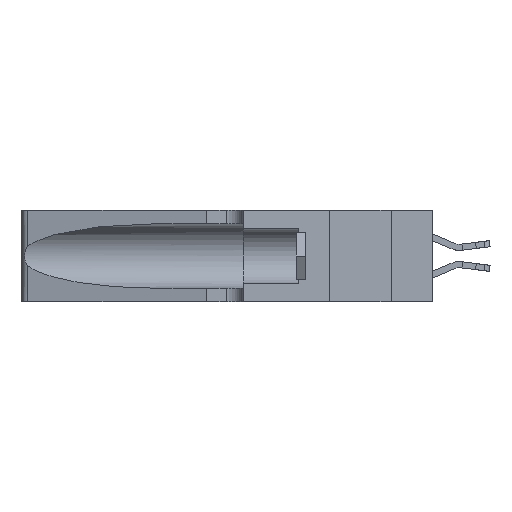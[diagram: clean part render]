
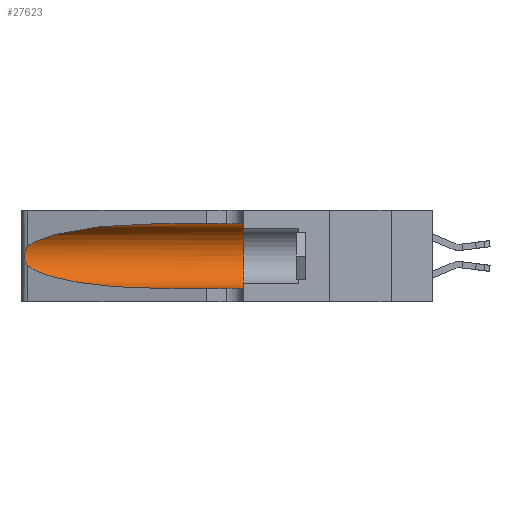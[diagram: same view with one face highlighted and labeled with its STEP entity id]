
A CAD part, left-side view. The second image highlights one B-rep face of the part: STEP entity #27623.
In plain terms, the highlighted cylindrical face has radius 3.308 mm (diameter 6.617 mm), a partial arc.
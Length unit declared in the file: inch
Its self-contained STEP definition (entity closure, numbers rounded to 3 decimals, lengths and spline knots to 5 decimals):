
#132 = CARTESIAN_POINT ( 'NONE',  ( 0.18966, 0.96281, 0.31525 ) ) ;
#293 = CARTESIAN_POINT ( 'NONE',  ( 0.1305, 0.35, 0.05475 ) ) ;
#329 = DIRECTION ( 'NONE',  ( 0., 1., 0. ) ) ;
#581 = B_SPLINE_CURVE_WITH_KNOTS ( 'NONE', 3,
 ( #30651, #11926, #3813, #22719, #6568, #25376, #9314, #28063, #12038, #30769, #14744, #33465, #17447, #1171 ),
 .UNSPECIFIED., .F., .F.,
 ( 4, 2, 2, 2, 2, 2, 4 ),
 ( 0., 0.00027, 0.00053, 0.00107, 0.0016, 0.00187, 0.00214 ),
 .UNSPECIFIED. ) ;
#1171 = CARTESIAN_POINT ( 'NONE',  ( 0.25487, 1.22718, 0.14631 ) ) ;
#1228 = ORIENTED_EDGE ( 'NONE', *, *, #17873, .T. ) ;
#1542 = EDGE_CURVE ( 'NONE', #30085, #18338, #31185, .T. ) ;
#2162 = LINE ( 'NONE', #15308, #22904 ) ;
#2334 = EDGE_CURVE ( 'NONE', #8358, #18338, #21103, .T. ) ;
#2861 = CARTESIAN_POINT ( 'NONE',  ( 0.25487, 1.22718, 0.14631 ) ) ;
#3148 = ORIENTED_EDGE ( 'NONE', *, *, #9684, .T. ) ;
#3813 = CARTESIAN_POINT ( 'NONE',  ( 0.25639, 1.23184, 0.21858 ) ) ;
#4668 = DIRECTION ( 'NONE',  ( 0., -1., 0. ) ) ;
#5190 = DIRECTION ( 'NONE',  ( 0., -1., 0. ) ) ;
#6568 = CARTESIAN_POINT ( 'NONE',  ( 0.25854, 1.2359, 0.20912 ) ) ;
#6579 = CARTESIAN_POINT ( 'NONE',  ( 0.1305, 0.72297, 0.31525 ) ) ;
#7106 = EDGE_CURVE ( 'NONE', #12279, #8358, #2162, .T. ) ;
#7494 = ORIENTED_EDGE ( 'NONE', *, *, #7106, .F. ) ;
#8358 = VERTEX_POINT ( 'NONE', #23224 ) ;
#8419 = CARTESIAN_POINT ( 'NONE',  ( 0.2373, 1.15595, 0.28018 ) ) ;
#9314 = CARTESIAN_POINT ( 'NONE',  ( 0.26075, 1.23896, 0.19203 ) ) ;
#9684 = EDGE_CURVE ( 'NONE', #25313, #30085, #19503, .T. ) ;
#9974 = ORIENTED_EDGE ( 'NONE', *, *, #33260, .T. ) ;
#10244 = ORIENTED_EDGE ( 'NONE', *, *, #1542, .T. ) ;
#11926 = CARTESIAN_POINT ( 'NONE',  ( 0.25555, 1.22994, 0.2215 ) ) ;
#12038 = CARTESIAN_POINT ( 'NONE',  ( 0.26017, 1.23833, 0.17102 ) ) ;
#12279 = VERTEX_POINT ( 'NONE', #6579 ) ;
#12888 = CARTESIAN_POINT ( 'NONE',  ( 0.1305, 1.61858, 0.185 ) ) ;
#13805 = ORIENTED_EDGE ( 'NONE', *, *, #2334, .F. ) ;
#14398 = CARTESIAN_POINT ( 'NONE',  ( 0.1305, 0.72297, 0.05475 ) ) ;
#14744 = CARTESIAN_POINT ( 'NONE',  ( 0.25789, 1.23486, 0.15765 ) ) ;
#15308 = CARTESIAN_POINT ( 'NONE',  ( 0.1305, 1.61858, 0.31525 ) ) ;
#16062 = AXIS2_PLACEMENT_3D ( 'NONE', #12888, #4668, #28899 ) ;
#16620 = CARTESIAN_POINT ( 'NONE',  ( 0.1305, 0.35, 0.185 ) ) ;
#16964 = VECTOR ( 'NONE', #5190, 39.37008 ) ;
#17383 = CARTESIAN_POINT ( 'NONE',  ( 0.2373, 1.15595, 0.08982 ) ) ;
#17447 = CARTESIAN_POINT ( 'NONE',  ( 0.25555, 1.22993, 0.14849 ) ) ;
#17873 = EDGE_CURVE ( 'NONE', #28362, #25313, #581, .T. ) ;
#18020 = DIRECTION ( 'NONE',  ( 0., -1., 0. ) ) ;
#18338 = VERTEX_POINT ( 'NONE', #293 ) ;
#19322 = DIRECTION ( 'NONE',  ( 0., 0., 1. ) ) ;
#19503 =( BOUNDED_CURVE ( )  B_SPLINE_CURVE ( 3, ( #20062, #17383, #33392, #22762 ),
 .UNSPECIFIED., .F., .F. ) 
 B_SPLINE_CURVE_WITH_KNOTS ( ( 4, 4 ),
 ( 3.44316, 4.71239 ),
 .UNSPECIFIED. ) 
 CURVE ( )  GEOMETRIC_REPRESENTATION_ITEM ( )  RATIONAL_B_SPLINE_CURVE ( ( 1., 0.87, 0.87, 1. ) ) 
 REPRESENTATION_ITEM ( '' )  );
#19615 = AXIS2_PLACEMENT_3D ( 'NONE', #16620, #329, #19322 ) ;
#20062 = CARTESIAN_POINT ( 'NONE',  ( 0.25487, 1.22718, 0.14631 ) ) ;
#20161 = FACE_OUTER_BOUND ( 'NONE', #24514, .T. ) ;
#21103 = CIRCLE ( 'NONE', #19615, 0.13025 ) ;
#22719 = CARTESIAN_POINT ( 'NONE',  ( 0.25787, 1.23484, 0.2124 ) ) ;
#22762 = CARTESIAN_POINT ( 'NONE',  ( 0.1305, 0.72297, 0.05475 ) ) ;
#22904 = VECTOR ( 'NONE', #18020, 39.37008 ) ;
#23224 = CARTESIAN_POINT ( 'NONE',  ( 0.1305, 0.35, 0.31525 ) ) ;
#23754 = CARTESIAN_POINT ( 'NONE',  ( 0.25487, 1.22718, 0.22369 ) ) ;
#24514 = EDGE_LOOP ( 'NONE', ( #9974, #1228, #3148, #10244, #13805, #7494 ) ) ;
#25313 = VERTEX_POINT ( 'NONE', #2861 ) ;
#25376 = CARTESIAN_POINT ( 'NONE',  ( 0.26018, 1.23835, 0.19895 ) ) ;
#27181 = CARTESIAN_POINT ( 'NONE',  ( 0.25487, 1.22718, 0.22369 ) ) ;
#27623 = ADVANCED_FACE ( 'NONE', ( #20161 ), #33550, .F. ) ;
#28063 = CARTESIAN_POINT ( 'NONE',  ( 0.26075, 1.23896, 0.178 ) ) ;
#28362 = VERTEX_POINT ( 'NONE', #23754 ) ;
#28899 = DIRECTION ( 'NONE',  ( 0., 0., -1. ) ) ;
#30085 = VERTEX_POINT ( 'NONE', #14398 ) ;
#30433 =( BOUNDED_CURVE ( )  B_SPLINE_CURVE ( 3, ( #32463, #132, #8419, #27181 ),
 .UNSPECIFIED., .F., .T. ) 
 B_SPLINE_CURVE_WITH_KNOTS ( ( 4, 4 ),
 ( 1.5708, 2.84003 ),
 .UNSPECIFIED. ) 
 CURVE ( )  GEOMETRIC_REPRESENTATION_ITEM ( )  RATIONAL_B_SPLINE_CURVE ( ( 1., 0.87, 0.87, 1. ) ) 
 REPRESENTATION_ITEM ( '' )  );
#30651 = CARTESIAN_POINT ( 'NONE',  ( 0.25487, 1.22718, 0.22369 ) ) ;
#30769 = CARTESIAN_POINT ( 'NONE',  ( 0.25856, 1.23593, 0.16098 ) ) ;
#31185 = LINE ( 'NONE', #34691, #16964 ) ;
#32463 = CARTESIAN_POINT ( 'NONE',  ( 0.1305, 0.72297, 0.31525 ) ) ;
#33260 = EDGE_CURVE ( 'NONE', #12279, #28362, #30433, .T. ) ;
#33392 = CARTESIAN_POINT ( 'NONE',  ( 0.18966, 0.96281, 0.05475 ) ) ;
#33465 = CARTESIAN_POINT ( 'NONE',  ( 0.25639, 1.23186, 0.15144 ) ) ;
#33550 = CYLINDRICAL_SURFACE ( 'NONE', #16062, 0.13025 ) ;
#34691 = CARTESIAN_POINT ( 'NONE',  ( 0.1305, 1.61858, 0.05475 ) ) ;
